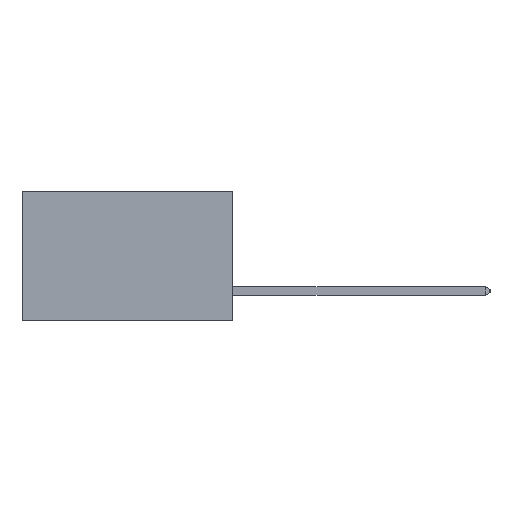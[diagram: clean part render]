
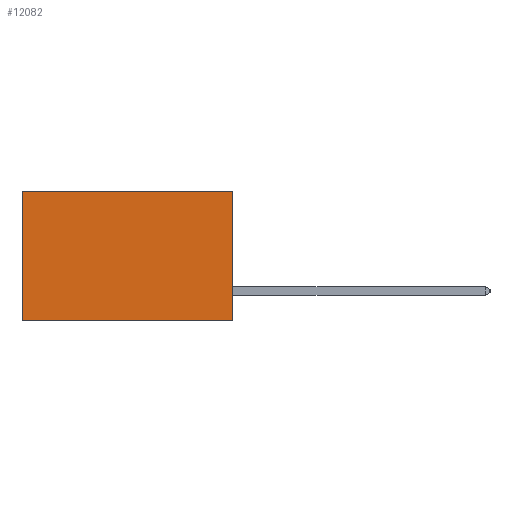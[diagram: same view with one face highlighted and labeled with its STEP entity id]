
A CAD part, left-side view. The second image highlights one B-rep face of the part: STEP entity #12082.
In plain terms, the highlighted planar face has unit normal (-1, 0, 0).
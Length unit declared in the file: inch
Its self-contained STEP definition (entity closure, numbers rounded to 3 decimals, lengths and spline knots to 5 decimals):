
#828 = CARTESIAN_POINT ( 'NONE',  ( 0.2875, 0.6, 0. ) ) ;
#1577 = CARTESIAN_POINT ( 'NONE',  ( 0.2875, 0.6, -0.37 ) ) ;
#2010 = ORIENTED_EDGE ( 'NONE', *, *, #30105, .T. ) ;
#4447 = ORIENTED_EDGE ( 'NONE', *, *, #21885, .F. ) ;
#6626 = VERTEX_POINT ( 'NONE', #11985 ) ;
#7130 = DIRECTION ( 'NONE',  ( 0., 0., -1. ) ) ;
#7992 = ORIENTED_EDGE ( 'NONE', *, *, #13330, .F. ) ;
#8154 = VERTEX_POINT ( 'NONE', #13829 ) ;
#9649 = CARTESIAN_POINT ( 'NONE',  ( 0.2875, 0., 0. ) ) ;
#10196 = LINE ( 'NONE', #9649, #29461 ) ;
#10597 = ORIENTED_EDGE ( 'NONE', *, *, #17118, .T. ) ;
#11081 = DIRECTION ( 'NONE',  ( 0., 1., 0. ) ) ;
#11985 = CARTESIAN_POINT ( 'NONE',  ( 0.2875, 0., 0. ) ) ;
#12082 = ADVANCED_FACE ( 'NONE', ( #21899 ), #12181, .F. ) ;
#12181 = PLANE ( 'NONE',  #14864 ) ;
#12295 = DIRECTION ( 'NONE',  ( 0., 0., -1. ) ) ;
#12299 = VECTOR ( 'NONE', #21007, 39.37008 ) ;
#12611 = VERTEX_POINT ( 'NONE', #1577 ) ;
#12935 = CARTESIAN_POINT ( 'NONE',  ( 0.2875, 0., -0.37 ) ) ;
#13084 = LINE ( 'NONE', #828, #12299 ) ;
#13330 = EDGE_CURVE ( 'NONE', #6626, #14217, #10196, .T. ) ;
#13603 = CARTESIAN_POINT ( 'NONE',  ( 0.2875, 0., 0. ) ) ;
#13829 = CARTESIAN_POINT ( 'NONE',  ( 0.2875, 0.6, 0. ) ) ;
#14217 = VERTEX_POINT ( 'NONE', #18592 ) ;
#14864 = AXIS2_PLACEMENT_3D ( 'NONE', #32301, #27377, #12295 ) ;
#17118 = EDGE_CURVE ( 'NONE', #6626, #8154, #31987, .T. ) ;
#18592 = CARTESIAN_POINT ( 'NONE',  ( 0.2875, 0., -0.37 ) ) ;
#18611 = VECTOR ( 'NONE', #11081, 39.37008 ) ;
#21007 = DIRECTION ( 'NONE',  ( 0., 0., -1. ) ) ;
#21885 = EDGE_CURVE ( 'NONE', #14217, #12611, #27493, .T. ) ;
#21899 = FACE_OUTER_BOUND ( 'NONE', #22991, .T. ) ;
#22991 = EDGE_LOOP ( 'NONE', ( #2010, #4447, #7992, #10597 ) ) ;
#25616 = DIRECTION ( 'NONE',  ( 0., 1., 0. ) ) ;
#27377 = DIRECTION ( 'NONE',  ( 1., 0., 0. ) ) ;
#27493 = LINE ( 'NONE', #12935, #32576 ) ;
#29461 = VECTOR ( 'NONE', #7130, 39.37008 ) ;
#30105 = EDGE_CURVE ( 'NONE', #8154, #12611, #13084, .T. ) ;
#31987 = LINE ( 'NONE', #13603, #18611 ) ;
#32301 = CARTESIAN_POINT ( 'NONE',  ( 0.2875, 0., 0. ) ) ;
#32576 = VECTOR ( 'NONE', #25616, 39.37008 ) ;
